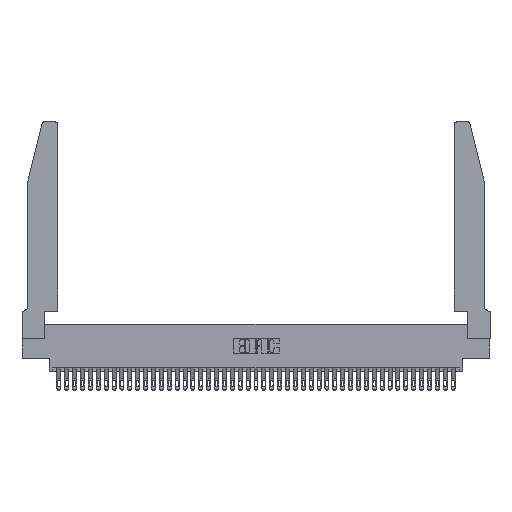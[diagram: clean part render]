
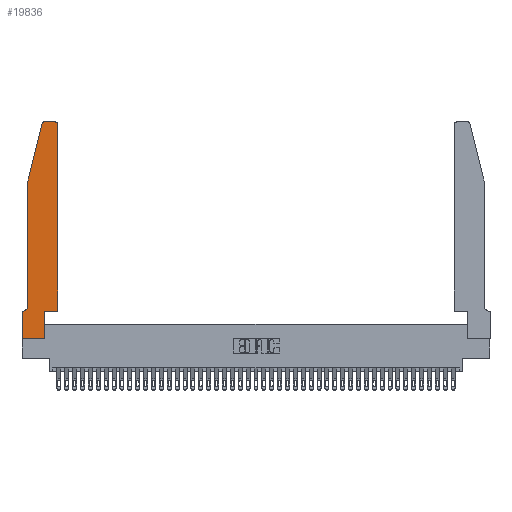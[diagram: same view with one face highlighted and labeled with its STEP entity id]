
A CAD part, top view. The second image highlights one B-rep face of the part: STEP entity #19836.
In plain terms, the highlighted planar face has unit normal (0, 0, 1).
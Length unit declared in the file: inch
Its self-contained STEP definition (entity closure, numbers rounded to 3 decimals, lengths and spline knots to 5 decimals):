
#26 = DIRECTION ( 'NONE',  ( -1., 0., 0. ) ) ;
#1552 = VERTEX_POINT ( 'NONE', #20295 ) ;
#1701 = LINE ( 'NONE', #33847, #36806 ) ;
#2283 = ORIENTED_EDGE ( 'NONE', *, *, #25685, .T. ) ;
#2593 = EDGE_CURVE ( 'NONE', #17476, #8830, #26632, .T. ) ;
#2764 = DIRECTION ( 'NONE',  ( 0., 0., 1. ) ) ;
#4068 = CARTESIAN_POINT ( 'NONE',  ( 0.284, 2.72, 0.37 ) ) ;
#4345 = CARTESIAN_POINT ( 'NONE',  ( 0., 0.35, 0.37 ) ) ;
#4496 = ORIENTED_EDGE ( 'NONE', *, *, #5340, .T. ) ;
#4893 = LINE ( 'NONE', #30805, #18180 ) ;
#5340 = EDGE_CURVE ( 'NONE', #8830, #26213, #17797, .T. ) ;
#5959 = VECTOR ( 'NONE', #37168, 39.37008 ) ;
#6439 = CARTESIAN_POINT ( 'NONE',  ( 0.0755, 0.42, 0.37 ) ) ;
#7439 = DIRECTION ( 'NONE',  ( 0., 0., 1. ) ) ;
#7538 = CARTESIAN_POINT ( 'NONE',  ( 0.25487, 2.72718, 0.37 ) ) ;
#7610 = CARTESIAN_POINT ( 'NONE',  ( 0., 0., 0.37 ) ) ;
#7676 = VERTEX_POINT ( 'NONE', #26568 ) ;
#7926 = DIRECTION ( 'NONE',  ( -0.239, -0.971, 0. ) ) ;
#8803 = VECTOR ( 'NONE', #41811, 39.37008 ) ;
#8830 = VERTEX_POINT ( 'NONE', #36599 ) ;
#9182 = EDGE_CURVE ( 'NONE', #31093, #29823, #9488, .T. ) ;
#9488 = CIRCLE ( 'NONE', #10602, 0.03 ) ;
#9905 = ORIENTED_EDGE ( 'NONE', *, *, #34099, .T. ) ;
#9909 = CARTESIAN_POINT ( 'NONE',  ( 0.2605, 2.75, 0.37 ) ) ;
#10602 = AXIS2_PLACEMENT_3D ( 'NONE', #4068, #7439, #41427 ) ;
#10838 = ORIENTED_EDGE ( 'NONE', *, *, #17043, .T. ) ;
#11555 = CARTESIAN_POINT ( 'NONE',  ( 0.2865, 0.35, 0.37 ) ) ;
#11963 = CARTESIAN_POINT ( 'NONE',  ( 0.4205, 2.72, 0.37 ) ) ;
#13132 = CARTESIAN_POINT ( 'NONE',  ( 0., 0., 0.37 ) ) ;
#15113 = CARTESIAN_POINT ( 'NONE',  ( 0., 0.35, 0.37 ) ) ;
#15150 = EDGE_CURVE ( 'NONE', #7676, #17476, #4893, .T. ) ;
#15468 = FACE_OUTER_BOUND ( 'NONE', #35453, .T. ) ;
#15628 = AXIS2_PLACEMENT_3D ( 'NONE', #16261, #43528, #33382 ) ;
#16261 = CARTESIAN_POINT ( 'NONE',  ( 0.0055, 0.42, 0.37 ) ) ;
#16368 = LINE ( 'NONE', #13132, #41979 ) ;
#17043 = EDGE_CURVE ( 'NONE', #29823, #7676, #33317, .T. ) ;
#17476 = VERTEX_POINT ( 'NONE', #6439 ) ;
#17797 = LINE ( 'NONE', #27715, #41781 ) ;
#17826 = CARTESIAN_POINT ( 'NONE',  ( 0.2865, 0.35, 0.37 ) ) ;
#18030 = LINE ( 'NONE', #9909, #28180 ) ;
#18099 = DIRECTION ( 'NONE',  ( 1., 0., 0. ) ) ;
#18180 = VECTOR ( 'NONE', #38538, 39.37008 ) ;
#18379 = CARTESIAN_POINT ( 'NONE',  ( 0.0755, 2., 0.37 ) ) ;
#19836 = ADVANCED_FACE ( 'NONE', ( #15468 ), #35944, .T. ) ;
#19914 = CARTESIAN_POINT ( 'NONE',  ( 0., 0., 0.37 ) ) ;
#20008 = VECTOR ( 'NONE', #7926, 39.37008 ) ;
#20040 = LINE ( 'NONE', #17826, #8803 ) ;
#20295 = CARTESIAN_POINT ( 'NONE',  ( 0.2865, 0., 0.37 ) ) ;
#20696 = CARTESIAN_POINT ( 'NONE',  ( 0.284, 2.75, 0.37 ) ) ;
#21081 = ORIENTED_EDGE ( 'NONE', *, *, #15150, .T. ) ;
#21124 = LINE ( 'NONE', #35087, #41696 ) ;
#21291 = DIRECTION ( 'NONE',  ( -1., 0., 0. ) ) ;
#22264 = DIRECTION ( 'NONE',  ( 0., 0., 1. ) ) ;
#22292 = EDGE_CURVE ( 'NONE', #34966, #1552, #16368, .T. ) ;
#22657 = VERTEX_POINT ( 'NONE', #34394 ) ;
#23254 = EDGE_CURVE ( 'NONE', #37750, #35212, #21124, .T. ) ;
#25456 = AXIS2_PLACEMENT_3D ( 'NONE', #15113, #22264, #38807 ) ;
#25685 = EDGE_CURVE ( 'NONE', #34736, #22657, #33331, .T. ) ;
#26213 = VERTEX_POINT ( 'NONE', #4345 ) ;
#26568 = CARTESIAN_POINT ( 'NONE',  ( 0.0755, 2., 0.37 ) ) ;
#26632 = CIRCLE ( 'NONE', #15628, 0.07 ) ;
#27715 = CARTESIAN_POINT ( 'NONE',  ( 0.0755, 0.35, 0.37 ) ) ;
#28180 = VECTOR ( 'NONE', #26, 39.37008 ) ;
#28998 = EDGE_CURVE ( 'NONE', #35212, #34736, #1701, .T. ) ;
#29823 = VERTEX_POINT ( 'NONE', #7538 ) ;
#30733 = DIRECTION ( 'NONE',  ( 0., 1., 0. ) ) ;
#30805 = CARTESIAN_POINT ( 'NONE',  ( 0.0755, 2., 0.37 ) ) ;
#31093 = VERTEX_POINT ( 'NONE', #20696 ) ;
#31874 = EDGE_CURVE ( 'NONE', #26213, #34966, #40063, .T. ) ;
#33317 = LINE ( 'NONE', #18379, #20008 ) ;
#33331 = CIRCLE ( 'NONE', #37943, 0.03 ) ;
#33382 = DIRECTION ( 'NONE',  ( -1., 0., 0. ) ) ;
#33527 = DIRECTION ( 'NONE',  ( 1., 0., 0. ) ) ;
#33847 = CARTESIAN_POINT ( 'NONE',  ( 0.4505, 0.35, 0.37 ) ) ;
#34099 = EDGE_CURVE ( 'NONE', #22657, #31093, #18030, .T. ) ;
#34394 = CARTESIAN_POINT ( 'NONE',  ( 0.4205, 2.75, 0.37 ) ) ;
#34736 = VERTEX_POINT ( 'NONE', #43417 ) ;
#34966 = VERTEX_POINT ( 'NONE', #7610 ) ;
#35087 = CARTESIAN_POINT ( 'NONE',  ( 0.4505, 0.35, 0.37 ) ) ;
#35188 = ORIENTED_EDGE ( 'NONE', *, *, #31874, .T. ) ;
#35212 = VERTEX_POINT ( 'NONE', #39415 ) ;
#35229 = ORIENTED_EDGE ( 'NONE', *, *, #22292, .T. ) ;
#35453 = EDGE_LOOP ( 'NONE', ( #9905, #39119, #10838, #21081, #42378, #4496, #35188, #35229, #40471, #39898, #41723, #2283 ) ) ;
#35944 = PLANE ( 'NONE',  #25456 ) ;
#36525 = DIRECTION ( 'NONE',  ( 1., 0., 0. ) ) ;
#36599 = CARTESIAN_POINT ( 'NONE',  ( 0.0055, 0.35, 0.37 ) ) ;
#36806 = VECTOR ( 'NONE', #30733, 39.37008 ) ;
#37168 = DIRECTION ( 'NONE',  ( 0., -1., 0. ) ) ;
#37750 = VERTEX_POINT ( 'NONE', #11555 ) ;
#37943 = AXIS2_PLACEMENT_3D ( 'NONE', #11963, #2764, #36525 ) ;
#38538 = DIRECTION ( 'NONE',  ( 0., -1., 0. ) ) ;
#38807 = DIRECTION ( 'NONE',  ( 1., 0., 0. ) ) ;
#39119 = ORIENTED_EDGE ( 'NONE', *, *, #9182, .T. ) ;
#39415 = CARTESIAN_POINT ( 'NONE',  ( 0.4505, 0.35, 0.37 ) ) ;
#39898 = ORIENTED_EDGE ( 'NONE', *, *, #23254, .T. ) ;
#40063 = LINE ( 'NONE', #19914, #5959 ) ;
#40471 = ORIENTED_EDGE ( 'NONE', *, *, #43513, .T. ) ;
#41427 = DIRECTION ( 'NONE',  ( 1., 0., 0. ) ) ;
#41696 = VECTOR ( 'NONE', #18099, 39.37008 ) ;
#41723 = ORIENTED_EDGE ( 'NONE', *, *, #28998, .T. ) ;
#41781 = VECTOR ( 'NONE', #21291, 39.37008 ) ;
#41811 = DIRECTION ( 'NONE',  ( 0., 1., 0. ) ) ;
#41979 = VECTOR ( 'NONE', #33527, 39.37008 ) ;
#42378 = ORIENTED_EDGE ( 'NONE', *, *, #2593, .T. ) ;
#43417 = CARTESIAN_POINT ( 'NONE',  ( 0.4505, 2.72, 0.37 ) ) ;
#43513 = EDGE_CURVE ( 'NONE', #1552, #37750, #20040, .T. ) ;
#43528 = DIRECTION ( 'NONE',  ( 0., 0., -1. ) ) ;
